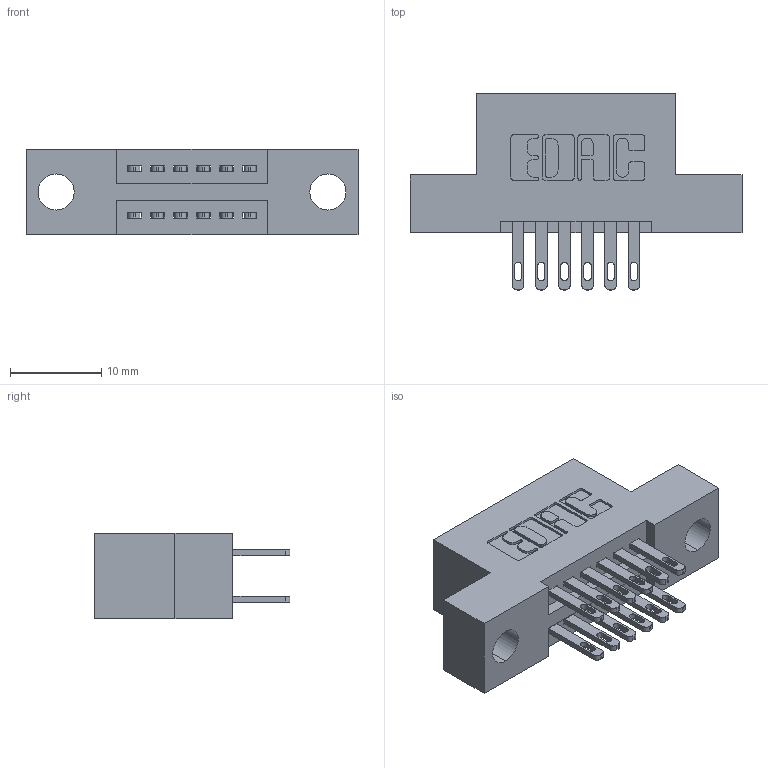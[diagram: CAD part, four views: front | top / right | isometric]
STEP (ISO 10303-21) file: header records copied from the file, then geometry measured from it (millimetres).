
FILE_DESCRIPTION (( 'STEP AP203' ), '1' );
FILE_NAME ('345-012-500-204.STEP', '2021-05-19T15:37:31', ( '' ), ( '' ), 'SwSTEP 2.0', 'SolidWorks 2020', '' );
FILE_SCHEMA (( 'CONFIG_CONTROL_DESIGN' ));
Length unit declared in the file: inch
Products named in the file (3): 345-292-001_345-293-100; 345 Part_Flush Mounting Lugs - 0.156 Dia-TI; 345-012-500-204
Assembly tree (13 placements, depth 2):
  345-012-500-204
    345 Part_Flush Mounting Lugs - 0.156 Dia-TI
    345-292-001_345-293-100  x12
Bounding box: 36.45 x 21.51 x 9.4 mm (x, y, z)
Volume: 3137.2 mm3; surface area: 3914.1 mm2
Topology: 13 solids, 13 shells, 692 faces, 2069 edges, 1378 vertices
Faces by surface type: plane 418, cylinder 274
Entity records: 9903 total; most frequent: CARTESIAN_POINT 1698, ORIENTED_EDGE 1630, DIRECTION 1543, EDGE_CURVE 815, LINE 655, VECTOR 655, VERTEX_POINT 542, AXIS2_PLACEMENT_3D 444
